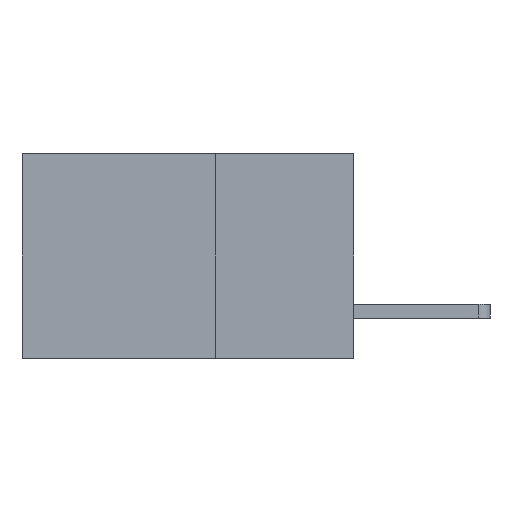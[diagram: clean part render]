
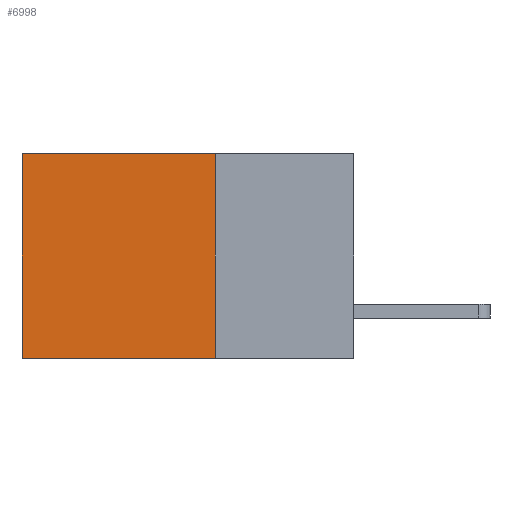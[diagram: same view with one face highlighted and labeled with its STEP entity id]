
A CAD part, left-side view. The second image highlights one B-rep face of the part: STEP entity #6998.
In plain terms, the highlighted planar face has unit normal (-1, 0, 0).
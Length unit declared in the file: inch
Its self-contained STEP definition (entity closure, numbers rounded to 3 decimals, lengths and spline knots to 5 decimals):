
#100 = VECTOR ( 'NONE', #3434, 39.37008 ) ;
#424 = LINE ( 'NONE', #470, #100 ) ;
#450 = EDGE_CURVE ( 'NONE', #3626, #7010, #2539, .T. ) ;
#470 = CARTESIAN_POINT ( 'NONE',  ( 0.2875, 0.25, -0.37 ) ) ;
#724 = CARTESIAN_POINT ( 'NONE',  ( 0.2875, 0.6, -0.37 ) ) ;
#927 = ORIENTED_EDGE ( 'NONE', *, *, #450, .T. ) ;
#1461 = LINE ( 'NONE', #2021, #3822 ) ;
#1776 = ORIENTED_EDGE ( 'NONE', *, *, #7860, .F. ) ;
#1890 = CARTESIAN_POINT ( 'NONE',  ( 0.2875, 0.6, 0. ) ) ;
#2021 = CARTESIAN_POINT ( 'NONE',  ( 0.2875, 0.25, 0. ) ) ;
#2137 = PLANE ( 'NONE',  #8363 ) ;
#2508 = CARTESIAN_POINT ( 'NONE',  ( 0.2875, 0.6, 0. ) ) ;
#2539 = LINE ( 'NONE', #1890, #5418 ) ;
#2663 = DIRECTION ( 'NONE',  ( 0., 0., -1. ) ) ;
#2667 = VECTOR ( 'NONE', #2663, 39.37008 ) ;
#2946 = EDGE_CURVE ( 'NONE', #6311, #3626, #1461, .T. ) ;
#3434 = DIRECTION ( 'NONE',  ( 0., 1., 0. ) ) ;
#3626 = VERTEX_POINT ( 'NONE', #2508 ) ;
#3749 = ORIENTED_EDGE ( 'NONE', *, *, #2946, .T. ) ;
#3822 = VECTOR ( 'NONE', #7866, 39.37008 ) ;
#3879 = DIRECTION ( 'NONE',  ( 0., 0., -1. ) ) ;
#4101 = LINE ( 'NONE', #5655, #2667 ) ;
#5073 = FACE_OUTER_BOUND ( 'NONE', #5893, .T. ) ;
#5418 = VECTOR ( 'NONE', #3879, 39.37008 ) ;
#5655 = CARTESIAN_POINT ( 'NONE',  ( 0.2875, 0.25, 0. ) ) ;
#5682 = CARTESIAN_POINT ( 'NONE',  ( 0.2875, 0.25, 0. ) ) ;
#5729 = DIRECTION ( 'NONE',  ( 0., 0., -1. ) ) ;
#5817 = CARTESIAN_POINT ( 'NONE',  ( 0.2875, 0.25, -0.37 ) ) ;
#5893 = EDGE_LOOP ( 'NONE', ( #927, #7385, #1776, #3749 ) ) ;
#6311 = VERTEX_POINT ( 'NONE', #5682 ) ;
#6484 = DIRECTION ( 'NONE',  ( 1., 0., 0. ) ) ;
#6998 = ADVANCED_FACE ( 'NONE', ( #5073 ), #2137, .F. ) ;
#7010 = VERTEX_POINT ( 'NONE', #724 ) ;
#7385 = ORIENTED_EDGE ( 'NONE', *, *, #9262, .F. ) ;
#7860 = EDGE_CURVE ( 'NONE', #6311, #8002, #4101, .T. ) ;
#7866 = DIRECTION ( 'NONE',  ( 0., 1., 0. ) ) ;
#7936 = CARTESIAN_POINT ( 'NONE',  ( 0.2875, 0.25, 0. ) ) ;
#8002 = VERTEX_POINT ( 'NONE', #5817 ) ;
#8363 = AXIS2_PLACEMENT_3D ( 'NONE', #7936, #6484, #5729 ) ;
#9262 = EDGE_CURVE ( 'NONE', #8002, #7010, #424, .T. ) ;
